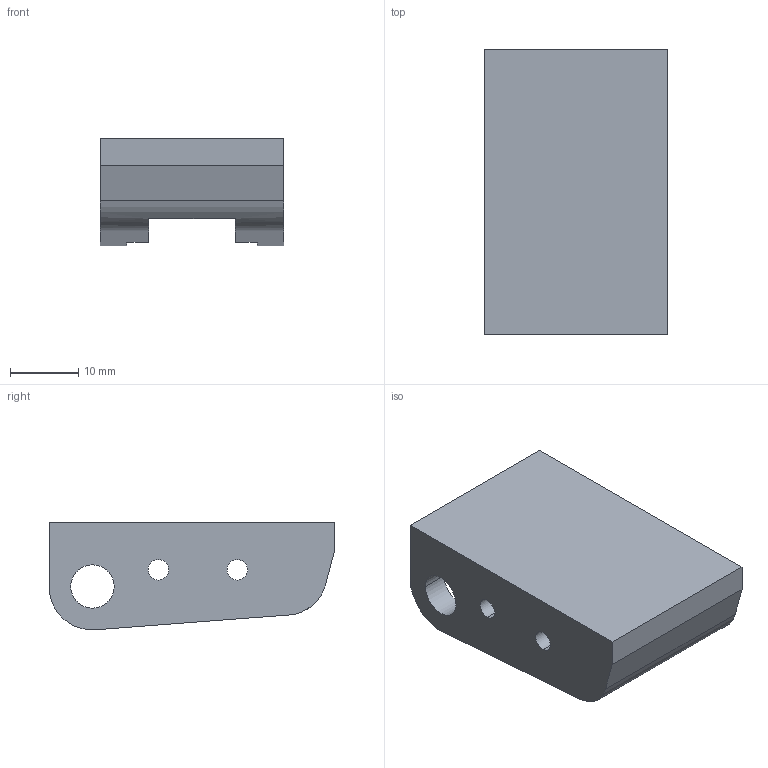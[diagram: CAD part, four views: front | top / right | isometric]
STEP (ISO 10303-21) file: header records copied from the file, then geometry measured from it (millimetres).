
FILE_DESCRIPTION (( 'STEP AP214' ), '1' );
FILE_NAME ('Thunderbolt_Mag_Well_Front.STEP', '2021-09-12T03:38:20', ( '' ), ( '' ), 'SwSTEP 2.0', 'SolidWorks 2020', '' );
FILE_SCHEMA (( 'AUTOMOTIVE_DESIGN' ));
Length unit declared in the file: millimetre
Products named in the file (1): Thunderbolt_Mag_Well_Front
Bounding box: 26.88 x 41.83 x 15.74 mm (x, y, z)
Volume: 11516.3 mm3; surface area: 4970.6 mm2
Topology: 1 solids, 1 shells, 27 faces, 77 edges, 52 vertices
Faces by surface type: plane 15, cylinder 12
Entity records: 943 total; most frequent: DIRECTION 159, CARTESIAN_POINT 157, ORIENTED_EDGE 154, EDGE_CURVE 77, AXIS2_PLACEMENT_3D 54, VERTEX_POINT 52, LINE 51, VECTOR 51
